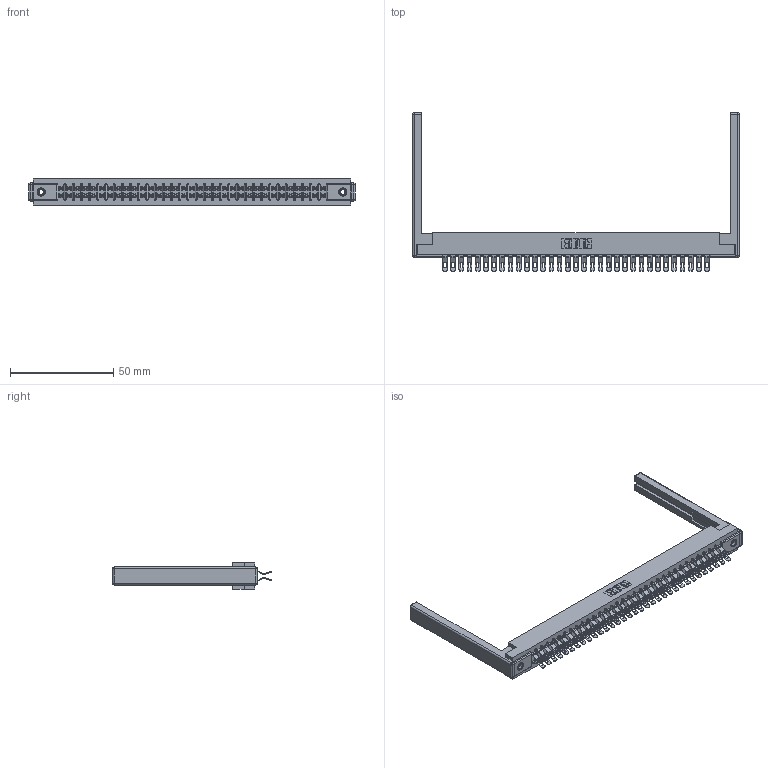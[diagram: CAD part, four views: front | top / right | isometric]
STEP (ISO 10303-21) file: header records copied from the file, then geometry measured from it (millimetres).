
FILE_DESCRIPTION (( 'STEP AP203' ), '1' );
FILE_NAME ('357-066-555-268.STEP', '2019-09-19T08:47:56', ( '' ), ( '' ), 'SwSTEP 2.0', 'SolidWorks 2016', '' );
FILE_SCHEMA (( 'CONFIG_CONTROL_DESIGN' ));
Length unit declared in the file: inch
Products named in the file (5): 307 Part_.156 Dia Mounting Holes; 345-250-001_345-250-001-102; 307-220-068; 307-290-001_555; 357-066-555-268
Assembly tree (71 placements, depth 2):
  357-066-555-268
    307 Part_.156 Dia Mounting Holes
    307-290-001_555  x66
    307-220-068  x2
    345-250-001_345-250-001-102  x2
Bounding box: 158.19 x 76.71 x 12.7 mm (x, y, z)
Volume: 21335.2 mm3; surface area: 25636.7 mm2
Topology: 71 solids, 71 shells, 4332 faces, 12659 edges, 8238 vertices
Faces by surface type: plane 2402, cylinder 1838, sphere 76, cone 12, torus 4
Entity records: 33752 total; most frequent: CARTESIAN_POINT 5506, ORIENTED_EDGE 5450, DIRECTION 5419, EDGE_CURVE 2725, LINE 2073, VECTOR 2073, VERTEX_POINT 1760, AXIS2_PLACEMENT_3D 1673
